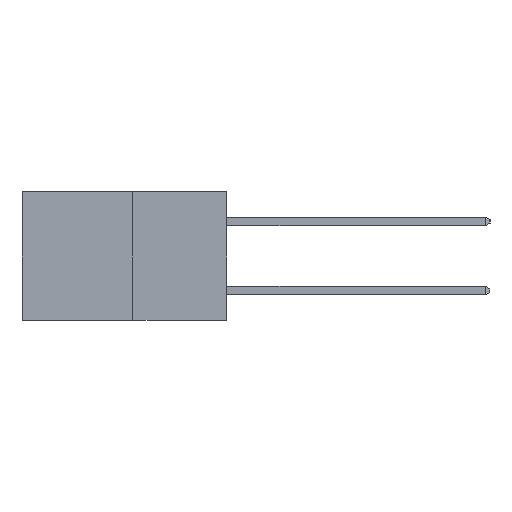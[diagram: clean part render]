
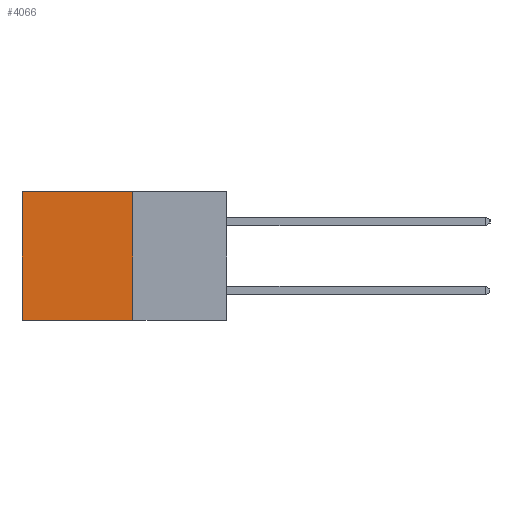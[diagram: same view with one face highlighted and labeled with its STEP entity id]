
A CAD part, left-side view. The second image highlights one B-rep face of the part: STEP entity #4066.
In plain terms, the highlighted planar face has unit normal (-1, 0, 0).
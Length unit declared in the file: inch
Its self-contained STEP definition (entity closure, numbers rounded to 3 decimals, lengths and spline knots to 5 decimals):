
#103 = AXIS2_PLACEMENT_3D ( 'NONE', #17275, #17111, #17035 ) ;
#850 = ORIENTED_EDGE ( 'NONE', *, *, #17123, .T. ) ;
#4066 = ADVANCED_FACE ( 'NONE', ( #11436 ), #18218, .F. ) ;
#4345 = VECTOR ( 'NONE', #7447, 39.37008 ) ;
#4352 = VERTEX_POINT ( 'NONE', #8719 ) ;
#4865 = EDGE_CURVE ( 'NONE', #8232, #6064, #13731, .T. ) ;
#5290 = EDGE_LOOP ( 'NONE', ( #850, #7944, #15545, #15469 ) ) ;
#6064 = VERTEX_POINT ( 'NONE', #7084 ) ;
#6335 = VERTEX_POINT ( 'NONE', #24269 ) ;
#7084 = CARTESIAN_POINT ( 'NONE',  ( 0.277, 0.59, -0.37 ) ) ;
#7447 = DIRECTION ( 'NONE',  ( 0., 1., 0. ) ) ;
#7930 = EDGE_CURVE ( 'NONE', #4352, #8232, #20310, .T. ) ;
#7944 = ORIENTED_EDGE ( 'NONE', *, *, #4865, .F. ) ;
#8232 = VERTEX_POINT ( 'NONE', #12322 ) ;
#8719 = CARTESIAN_POINT ( 'NONE',  ( 0.277, 0.27, 0. ) ) ;
#9337 = LINE ( 'NONE', #23450, #14924 ) ;
#10339 = VECTOR ( 'NONE', #22617, 39.37008 ) ;
#11436 = FACE_OUTER_BOUND ( 'NONE', #5290, .T. ) ;
#11793 = CARTESIAN_POINT ( 'NONE',  ( 0.277, 0.59, -0.37 ) ) ;
#12215 = VECTOR ( 'NONE', #23067, 39.37008 ) ;
#12246 = DIRECTION ( 'NONE',  ( 0., 1., 0. ) ) ;
#12322 = CARTESIAN_POINT ( 'NONE',  ( 0.277, 0.27, -0.37 ) ) ;
#13731 = LINE ( 'NONE', #15858, #4345 ) ;
#13962 = LINE ( 'NONE', #11793, #12215 ) ;
#14924 = VECTOR ( 'NONE', #12246, 39.37008 ) ;
#15469 = ORIENTED_EDGE ( 'NONE', *, *, #15895, .T. ) ;
#15545 = ORIENTED_EDGE ( 'NONE', *, *, #7930, .F. ) ;
#15858 = CARTESIAN_POINT ( 'NONE',  ( 0.277, 0.27, -0.37 ) ) ;
#15895 = EDGE_CURVE ( 'NONE', #4352, #6335, #9337, .T. ) ;
#17035 = DIRECTION ( 'NONE',  ( 0., 0., -1. ) ) ;
#17111 = DIRECTION ( 'NONE',  ( 1., 0., 0. ) ) ;
#17123 = EDGE_CURVE ( 'NONE', #6335, #6064, #13962, .T. ) ;
#17275 = CARTESIAN_POINT ( 'NONE',  ( 0.277, 0.27, -0.37 ) ) ;
#18218 = PLANE ( 'NONE',  #103 ) ;
#20310 = LINE ( 'NONE', #22803, #10339 ) ;
#22617 = DIRECTION ( 'NONE',  ( 0., 0., -1. ) ) ;
#22803 = CARTESIAN_POINT ( 'NONE',  ( 0.277, 0.27, -0.37 ) ) ;
#23067 = DIRECTION ( 'NONE',  ( 0., 0., -1. ) ) ;
#23450 = CARTESIAN_POINT ( 'NONE',  ( 0.277, 0.27, 0. ) ) ;
#24269 = CARTESIAN_POINT ( 'NONE',  ( 0.277, 0.59, 0. ) ) ;
